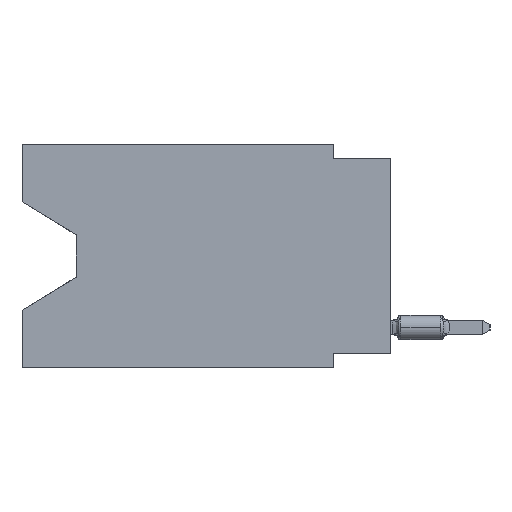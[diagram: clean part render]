
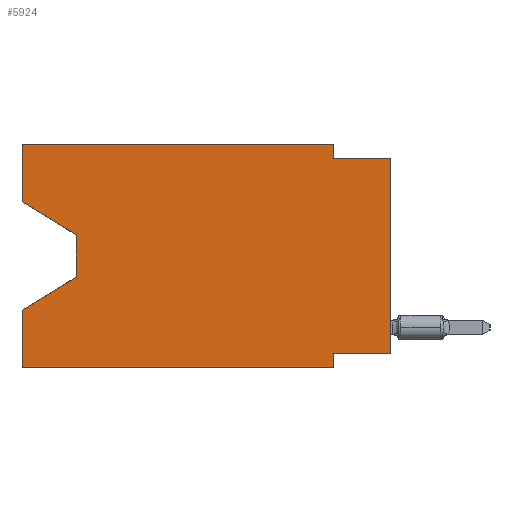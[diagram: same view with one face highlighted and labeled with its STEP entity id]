
A CAD part, left-side view. The second image highlights one B-rep face of the part: STEP entity #5924.
In plain terms, the highlighted planar face has unit normal (-1, 0, 0).
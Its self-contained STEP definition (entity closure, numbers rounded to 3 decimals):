
#409 = DIRECTION ( 'NONE',  ( 0., 0., 1. ) ) ;
#781 = LINE ( 'NONE', #9489, #10258 ) ;
#1089 = DIRECTION ( 'NONE',  ( 0., 0., 1. ) ) ;
#1157 = ORIENTED_EDGE ( 'NONE', *, *, #36903, .T. ) ;
#1438 = DIRECTION ( 'NONE',  ( 0., 0., -1. ) ) ;
#1737 = CARTESIAN_POINT ( 'NONE',  ( 0., 16.383, 0. ) ) ;
#2980 = EDGE_CURVE ( 'NONE', #29276, #5046, #32012, .T. ) ;
#3544 = CARTESIAN_POINT ( 'NONE',  ( 0., 13.97, -4.013 ) ) ;
#3545 = VECTOR ( 'NONE', #17278, 1000. ) ;
#4232 = ORIENTED_EDGE ( 'NONE', *, *, #23665, .F. ) ;
#5046 = VERTEX_POINT ( 'NONE', #16234 ) ;
#5238 = VERTEX_POINT ( 'NONE', #18925 ) ;
#5352 = CARTESIAN_POINT ( 'NONE',  ( 0., 16.383, -9.906 ) ) ;
#5542 = LINE ( 'NONE', #5352, #25373 ) ;
#5724 = LINE ( 'NONE', #34908, #3545 ) ;
#5851 = ORIENTED_EDGE ( 'NONE', *, *, #11444, .T. ) ;
#5924 = ADVANCED_FACE ( 'NONE', ( #30232 ), #27378, .F. ) ;
#6734 = CARTESIAN_POINT ( 'NONE',  ( 0., 16.383, -2.546 ) ) ;
#6776 = CARTESIAN_POINT ( 'NONE',  ( 0., 16.383, -9.906 ) ) ;
#7341 = DIRECTION ( 'NONE',  ( 0., 0., -1. ) ) ;
#7360 = AXIS2_PLACEMENT_3D ( 'NONE', #24534, #30796, #31732 ) ;
#7383 = CARTESIAN_POINT ( 'NONE',  ( 0., 0., -9.271 ) ) ;
#7515 = CARTESIAN_POINT ( 'NONE',  ( 0., 2.54, 0. ) ) ;
#7630 = ORIENTED_EDGE ( 'NONE', *, *, #31736, .F. ) ;
#7961 = EDGE_CURVE ( 'NONE', #18125, #34983, #13367, .T. ) ;
#8561 = CARTESIAN_POINT ( 'NONE',  ( 0., 16.383, 0. ) ) ;
#9348 = EDGE_CURVE ( 'NONE', #30554, #10892, #5542, .T. ) ;
#9407 = LINE ( 'NONE', #24559, #25263 ) ;
#9451 = ORIENTED_EDGE ( 'NONE', *, *, #15035, .F. ) ;
#9489 = CARTESIAN_POINT ( 'NONE',  ( 0., 16.383, 0. ) ) ;
#9497 = EDGE_CURVE ( 'NONE', #5238, #14971, #5724, .T. ) ;
#9594 = CARTESIAN_POINT ( 'NONE',  ( 0., 16.383, -7.36 ) ) ;
#10258 = VECTOR ( 'NONE', #409, 1000. ) ;
#10892 = VERTEX_POINT ( 'NONE', #35049 ) ;
#11444 = EDGE_CURVE ( 'NONE', #18125, #14136, #12223, .T. ) ;
#11661 = ORIENTED_EDGE ( 'NONE', *, *, #9497, .T. ) ;
#12100 = EDGE_CURVE ( 'NONE', #5046, #10892, #21012, .T. ) ;
#12219 = VERTEX_POINT ( 'NONE', #19831 ) ;
#12223 = LINE ( 'NONE', #21138, #29392 ) ;
#12391 = DIRECTION ( 'NONE',  ( 0., -1., 0. ) ) ;
#12793 = DIRECTION ( 'NONE',  ( 0., 0., -1. ) ) ;
#13367 = LINE ( 'NONE', #21168, #23012 ) ;
#13483 = VERTEX_POINT ( 'NONE', #7515 ) ;
#13693 = CARTESIAN_POINT ( 'NONE',  ( 0., 0., -0.635 ) ) ;
#14136 = VERTEX_POINT ( 'NONE', #26221 ) ;
#14227 = EDGE_CURVE ( 'NONE', #12219, #21556, #30005, .T. ) ;
#14714 = EDGE_LOOP ( 'NONE', ( #5851, #32034, #11661, #7630, #33325, #28567, #17225, #1157, #35062, #9451, #4232, #20218 ) ) ;
#14904 = VECTOR ( 'NONE', #21278, 1000. ) ;
#14971 = VERTEX_POINT ( 'NONE', #9594 ) ;
#15035 = EDGE_CURVE ( 'NONE', #13483, #12219, #9407, .T. ) ;
#15040 = EDGE_CURVE ( 'NONE', #14136, #5238, #26671, .T. ) ;
#15506 = VECTOR ( 'NONE', #12391, 1000. ) ;
#16234 = CARTESIAN_POINT ( 'NONE',  ( 0., 2.54, -9.271 ) ) ;
#17225 = ORIENTED_EDGE ( 'NONE', *, *, #2980, .F. ) ;
#17278 = DIRECTION ( 'NONE',  ( 0., 0.855, -0.519 ) ) ;
#17599 = CARTESIAN_POINT ( 'NONE',  ( 0., 0., -9.271 ) ) ;
#18125 = VERTEX_POINT ( 'NONE', #6734 ) ;
#18925 = CARTESIAN_POINT ( 'NONE',  ( 0., 13.97, -5.893 ) ) ;
#19831 = CARTESIAN_POINT ( 'NONE',  ( 0., 2.54, -0.635 ) ) ;
#20136 = LINE ( 'NONE', #34919, #24957 ) ;
#20218 = ORIENTED_EDGE ( 'NONE', *, *, #7961, .F. ) ;
#20461 = VECTOR ( 'NONE', #1438, 1000. ) ;
#20512 = DIRECTION ( 'NONE',  ( 0., 0., 1. ) ) ;
#21012 = LINE ( 'NONE', #35407, #22745 ) ;
#21138 = CARTESIAN_POINT ( 'NONE',  ( 0., 16.383, -2.546 ) ) ;
#21168 = CARTESIAN_POINT ( 'NONE',  ( 0., 16.383, 0. ) ) ;
#21278 = DIRECTION ( 'NONE',  ( 0., -1., 0. ) ) ;
#21556 = VERTEX_POINT ( 'NONE', #13693 ) ;
#22745 = VECTOR ( 'NONE', #7341, 1000. ) ;
#23012 = VECTOR ( 'NONE', #1089, 1000. ) ;
#23665 = EDGE_CURVE ( 'NONE', #34983, #13483, #23969, .T. ) ;
#23969 = LINE ( 'NONE', #1737, #15506 ) ;
#24492 = CARTESIAN_POINT ( 'NONE',  ( 0., 0., -0.635 ) ) ;
#24534 = CARTESIAN_POINT ( 'NONE',  ( 0., 16.383, 0. ) ) ;
#24559 = CARTESIAN_POINT ( 'NONE',  ( 0., 2.54, 0. ) ) ;
#24957 = VECTOR ( 'NONE', #20512, 1000. ) ;
#25263 = VECTOR ( 'NONE', #12793, 1000. ) ;
#25373 = VECTOR ( 'NONE', #36797, 1000. ) ;
#26221 = CARTESIAN_POINT ( 'NONE',  ( 0., 13.97, -4.013 ) ) ;
#26671 = LINE ( 'NONE', #3544, #20461 ) ;
#27378 = PLANE ( 'NONE',  #7360 ) ;
#28089 = VECTOR ( 'NONE', #29158, 1000. ) ;
#28567 = ORIENTED_EDGE ( 'NONE', *, *, #12100, .F. ) ;
#29158 = DIRECTION ( 'NONE',  ( 0., 1., 0. ) ) ;
#29276 = VERTEX_POINT ( 'NONE', #7383 ) ;
#29392 = VECTOR ( 'NONE', #30557, 1000. ) ;
#30005 = LINE ( 'NONE', #24492, #14904 ) ;
#30232 = FACE_OUTER_BOUND ( 'NONE', #14714, .T. ) ;
#30554 = VERTEX_POINT ( 'NONE', #6776 ) ;
#30557 = DIRECTION ( 'NONE',  ( 0., -0.855, -0.519 ) ) ;
#30796 = DIRECTION ( 'NONE',  ( 1., 0., 0. ) ) ;
#31732 = DIRECTION ( 'NONE',  ( 0., 0., -1. ) ) ;
#31736 = EDGE_CURVE ( 'NONE', #30554, #14971, #781, .T. ) ;
#32012 = LINE ( 'NONE', #17599, #28089 ) ;
#32034 = ORIENTED_EDGE ( 'NONE', *, *, #15040, .T. ) ;
#33325 = ORIENTED_EDGE ( 'NONE', *, *, #9348, .T. ) ;
#34908 = CARTESIAN_POINT ( 'NONE',  ( 0., 13.97, -5.893 ) ) ;
#34919 = CARTESIAN_POINT ( 'NONE',  ( 0., 0., 0. ) ) ;
#34983 = VERTEX_POINT ( 'NONE', #8561 ) ;
#35049 = CARTESIAN_POINT ( 'NONE',  ( 0., 2.54, -9.906 ) ) ;
#35062 = ORIENTED_EDGE ( 'NONE', *, *, #14227, .F. ) ;
#35407 = CARTESIAN_POINT ( 'NONE',  ( 0., 2.54, -9.906 ) ) ;
#36797 = DIRECTION ( 'NONE',  ( 0., -1., 0. ) ) ;
#36903 = EDGE_CURVE ( 'NONE', #29276, #21556, #20136, .T. ) ;
